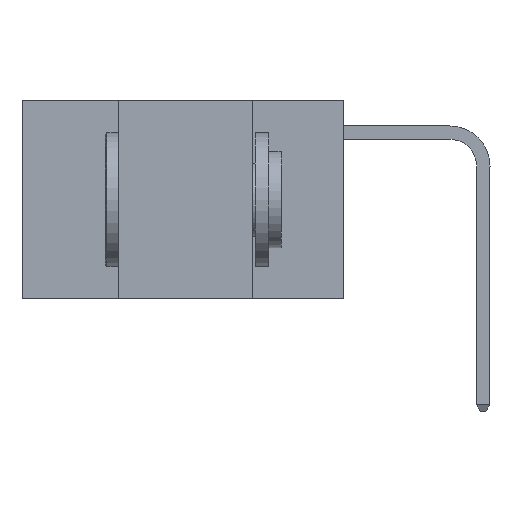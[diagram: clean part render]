
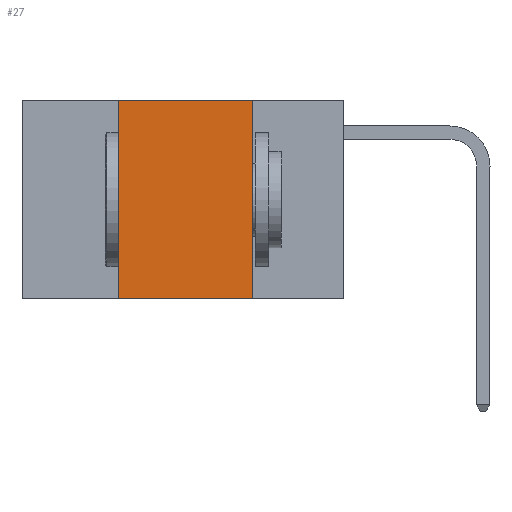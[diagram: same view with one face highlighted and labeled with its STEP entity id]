
A CAD part, left-side view. The second image highlights one B-rep face of the part: STEP entity #27.
In plain terms, the highlighted planar face has unit normal (-1, 0, 0).
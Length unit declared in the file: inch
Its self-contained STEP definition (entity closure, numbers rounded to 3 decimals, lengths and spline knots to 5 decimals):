
#22 = LINE ( 'NONE', #10557, #4416 ) ;
#27 = ADVANCED_FACE ( 'NONE', ( #5553 ), #9144, .F. ) ;
#72 = EDGE_CURVE ( 'NONE', #11016, #6582, #5124, .T. ) ;
#167 = VERTEX_POINT ( 'NONE', #2640 ) ;
#1746 = EDGE_LOOP ( 'NONE', ( #3448, #3474, #3608, #3724 ) ) ;
#1816 = VECTOR ( 'NONE', #3072, 39.37008 ) ;
#1858 = DIRECTION ( 'NONE',  ( 0., 0., 1. ) ) ;
#1974 = DIRECTION ( 'NONE',  ( 0., -1., 0. ) ) ;
#1993 = VERTEX_POINT ( 'NONE', #9088 ) ;
#1999 = CARTESIAN_POINT ( 'NONE',  ( 0., 0.42, -0.37 ) ) ;
#2103 = LINE ( 'NONE', #3098, #1816 ) ;
#2275 = CARTESIAN_POINT ( 'NONE',  ( 0., 0.6, -0.37 ) ) ;
#2640 = CARTESIAN_POINT ( 'NONE',  ( 0., 0.17, -0.37 ) ) ;
#3072 = DIRECTION ( 'NONE',  ( 0., -1., 0. ) ) ;
#3098 = CARTESIAN_POINT ( 'NONE',  ( 0., 0.6, 0. ) ) ;
#3448 = ORIENTED_EDGE ( 'NONE', *, *, #4363, .F. ) ;
#3474 = ORIENTED_EDGE ( 'NONE', *, *, #7277, .F. ) ;
#3608 = ORIENTED_EDGE ( 'NONE', *, *, #72, .F. ) ;
#3724 = ORIENTED_EDGE ( 'NONE', *, *, #4704, .T. ) ;
#4119 = LINE ( 'NONE', #2275, #4538 ) ;
#4363 = EDGE_CURVE ( 'NONE', #1993, #167, #22, .T. ) ;
#4416 = VECTOR ( 'NONE', #10357, 39.37008 ) ;
#4538 = VECTOR ( 'NONE', #1974, 39.37008 ) ;
#4704 = EDGE_CURVE ( 'NONE', #11016, #167, #4119, .T. ) ;
#5124 = LINE ( 'NONE', #7423, #5482 ) ;
#5362 = DIRECTION ( 'NONE',  ( 0., 0., -1. ) ) ;
#5482 = VECTOR ( 'NONE', #1858, 39.37008 ) ;
#5553 = FACE_OUTER_BOUND ( 'NONE', #1746, .T. ) ;
#5792 = AXIS2_PLACEMENT_3D ( 'NONE', #9255, #10377, #5362 ) ;
#6582 = VERTEX_POINT ( 'NONE', #11333 ) ;
#7277 = EDGE_CURVE ( 'NONE', #6582, #1993, #2103, .T. ) ;
#7423 = CARTESIAN_POINT ( 'NONE',  ( 0., 0.42, 0. ) ) ;
#9088 = CARTESIAN_POINT ( 'NONE',  ( 0., 0.17, 0. ) ) ;
#9144 = PLANE ( 'NONE',  #5792 ) ;
#9255 = CARTESIAN_POINT ( 'NONE',  ( 0., 0.6, 0. ) ) ;
#10357 = DIRECTION ( 'NONE',  ( 0., 0., -1. ) ) ;
#10377 = DIRECTION ( 'NONE',  ( 1., 0., 0. ) ) ;
#10557 = CARTESIAN_POINT ( 'NONE',  ( 0., 0.17, 0. ) ) ;
#11016 = VERTEX_POINT ( 'NONE', #1999 ) ;
#11333 = CARTESIAN_POINT ( 'NONE',  ( 0., 0.42, 0. ) ) ;
